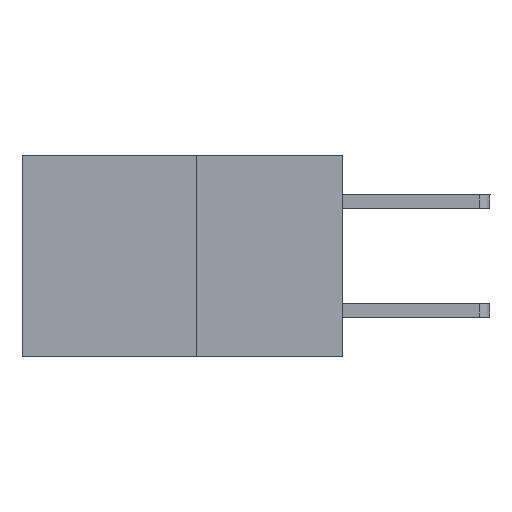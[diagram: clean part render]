
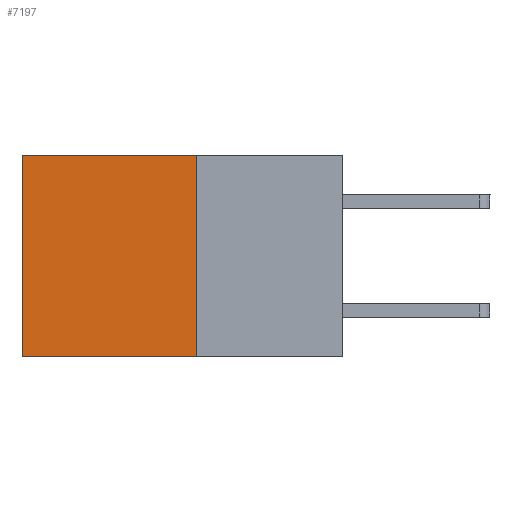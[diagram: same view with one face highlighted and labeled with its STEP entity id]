
A CAD part, left-side view. The second image highlights one B-rep face of the part: STEP entity #7197.
In plain terms, the highlighted planar face has unit normal (-1, 0, 0).
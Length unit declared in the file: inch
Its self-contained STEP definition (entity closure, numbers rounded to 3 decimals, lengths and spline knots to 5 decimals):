
#153 = DIRECTION ( 'NONE',  ( 0., 0., -1. ) ) ;
#1063 = VERTEX_POINT ( 'NONE', #2934 ) ;
#1741 = CARTESIAN_POINT ( 'NONE',  ( 0.277, 0.27, -0.37 ) ) ;
#1918 = DIRECTION ( 'NONE',  ( 0., 0., -1. ) ) ;
#2934 = CARTESIAN_POINT ( 'NONE',  ( 0.277, 0.27, 0. ) ) ;
#3239 = AXIS2_PLACEMENT_3D ( 'NONE', #9672, #12661, #6548 ) ;
#3427 = FACE_OUTER_BOUND ( 'NONE', #11873, .T. ) ;
#3801 = LINE ( 'NONE', #7815, #10061 ) ;
#4324 = CARTESIAN_POINT ( 'NONE',  ( 0.277, 0.59, -0.37 ) ) ;
#4649 = ORIENTED_EDGE ( 'NONE', *, *, #12847, .F. ) ;
#5185 = ORIENTED_EDGE ( 'NONE', *, *, #8744, .T. ) ;
#5427 = VERTEX_POINT ( 'NONE', #12440 ) ;
#5729 = DIRECTION ( 'NONE',  ( 0., 1., 0. ) ) ;
#5793 = CARTESIAN_POINT ( 'NONE',  ( 0.277, 0.27, -0.37 ) ) ;
#5849 = VERTEX_POINT ( 'NONE', #4324 ) ;
#6144 = ORIENTED_EDGE ( 'NONE', *, *, #10176, .T. ) ;
#6548 = DIRECTION ( 'NONE',  ( 0., 0., -1. ) ) ;
#6877 = VECTOR ( 'NONE', #5729, 39.37008 ) ;
#6909 = LINE ( 'NONE', #5793, #6877 ) ;
#7186 = CARTESIAN_POINT ( 'NONE',  ( 0.277, 0.27, -0.37 ) ) ;
#7197 = ADVANCED_FACE ( 'NONE', ( #3427 ), #8401, .F. ) ;
#7815 = CARTESIAN_POINT ( 'NONE',  ( 0.277, 0.27, 0. ) ) ;
#7948 = ORIENTED_EDGE ( 'NONE', *, *, #8067, .F. ) ;
#8067 = EDGE_CURVE ( 'NONE', #1063, #12851, #9245, .T. ) ;
#8401 = PLANE ( 'NONE',  #3239 ) ;
#8744 = EDGE_CURVE ( 'NONE', #5427, #5849, #12880, .T. ) ;
#9245 = LINE ( 'NONE', #7186, #10459 ) ;
#9383 = VECTOR ( 'NONE', #1918, 39.37008 ) ;
#9672 = CARTESIAN_POINT ( 'NONE',  ( 0.277, 0.27, -0.37 ) ) ;
#9949 = CARTESIAN_POINT ( 'NONE',  ( 0.277, 0.59, -0.37 ) ) ;
#10061 = VECTOR ( 'NONE', #11879, 39.37008 ) ;
#10176 = EDGE_CURVE ( 'NONE', #1063, #5427, #3801, .T. ) ;
#10459 = VECTOR ( 'NONE', #153, 39.37008 ) ;
#11873 = EDGE_LOOP ( 'NONE', ( #5185, #4649, #7948, #6144 ) ) ;
#11879 = DIRECTION ( 'NONE',  ( 0., 1., 0. ) ) ;
#12440 = CARTESIAN_POINT ( 'NONE',  ( 0.277, 0.59, 0. ) ) ;
#12661 = DIRECTION ( 'NONE',  ( 1., 0., 0. ) ) ;
#12847 = EDGE_CURVE ( 'NONE', #12851, #5849, #6909, .T. ) ;
#12851 = VERTEX_POINT ( 'NONE', #1741 ) ;
#12880 = LINE ( 'NONE', #9949, #9383 ) ;
